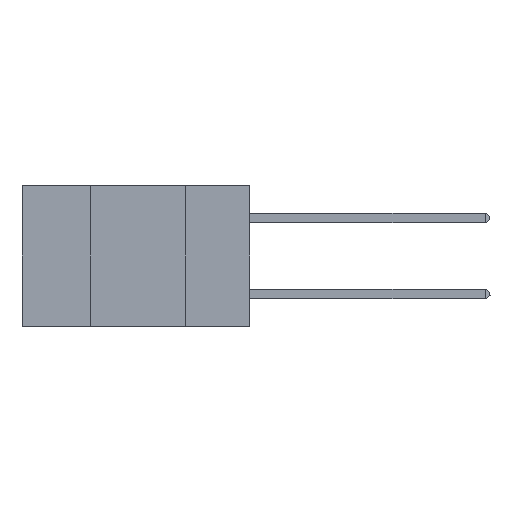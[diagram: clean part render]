
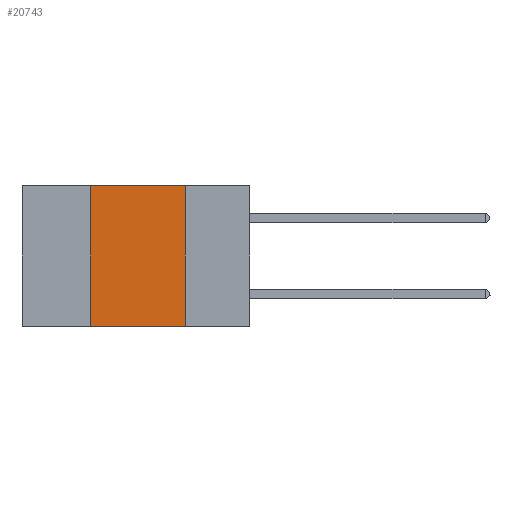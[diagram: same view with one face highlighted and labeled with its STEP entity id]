
A CAD part, left-side view. The second image highlights one B-rep face of the part: STEP entity #20743.
In plain terms, the highlighted planar face has unit normal (-1, 0, 0).
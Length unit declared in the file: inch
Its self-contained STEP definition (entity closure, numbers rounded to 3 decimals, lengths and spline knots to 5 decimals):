
#1144 = LINE ( 'NONE', #11175, #31647 ) ;
#2035 = CARTESIAN_POINT ( 'NONE',  ( 0., 0.6, 0. ) ) ;
#2526 = ORIENTED_EDGE ( 'NONE', *, *, #11613, .F. ) ;
#2671 = ORIENTED_EDGE ( 'NONE', *, *, #4228, .F. ) ;
#4228 = EDGE_CURVE ( 'NONE', #13115, #25626, #24204, .T. ) ;
#5015 = VECTOR ( 'NONE', #19980, 39.37008 ) ;
#5289 = ORIENTED_EDGE ( 'NONE', *, *, #32906, .F. ) ;
#5530 = EDGE_CURVE ( 'NONE', #36855, #7606, #1144, .T. ) ;
#5857 = EDGE_LOOP ( 'NONE', ( #2526, #2671, #5289, #28682 ) ) ;
#7606 = VERTEX_POINT ( 'NONE', #37992 ) ;
#8787 = LINE ( 'NONE', #32170, #28466 ) ;
#10577 = CARTESIAN_POINT ( 'NONE',  ( 0., 0.42, 0. ) ) ;
#11175 = CARTESIAN_POINT ( 'NONE',  ( 0., 0.6, -0.37 ) ) ;
#11613 = EDGE_CURVE ( 'NONE', #25626, #7606, #40055, .T. ) ;
#12917 = DIRECTION ( 'NONE',  ( 0., 0., 1. ) ) ;
#13115 = VERTEX_POINT ( 'NONE', #10577 ) ;
#13238 = FACE_OUTER_BOUND ( 'NONE', #5857, .T. ) ;
#13737 = VECTOR ( 'NONE', #39540, 39.37008 ) ;
#15308 = PLANE ( 'NONE',  #25705 ) ;
#17654 = DIRECTION ( 'NONE',  ( 0., -1., 0. ) ) ;
#18726 = DIRECTION ( 'NONE',  ( 1., 0., 0. ) ) ;
#19980 = DIRECTION ( 'NONE',  ( 0., 0., -1. ) ) ;
#20743 = ADVANCED_FACE ( 'NONE', ( #13238 ), #15308, .F. ) ;
#24204 = LINE ( 'NONE', #2035, #13737 ) ;
#25529 = CARTESIAN_POINT ( 'NONE',  ( 0., 0.42, -0.37 ) ) ;
#25626 = VERTEX_POINT ( 'NONE', #32098 ) ;
#25705 = AXIS2_PLACEMENT_3D ( 'NONE', #27922, #18726, #34688 ) ;
#27922 = CARTESIAN_POINT ( 'NONE',  ( 0., 0.6, 0. ) ) ;
#28466 = VECTOR ( 'NONE', #12917, 39.37008 ) ;
#28682 = ORIENTED_EDGE ( 'NONE', *, *, #5530, .T. ) ;
#29322 = CARTESIAN_POINT ( 'NONE',  ( 0., 0.17, 0. ) ) ;
#31647 = VECTOR ( 'NONE', #17654, 39.37008 ) ;
#32098 = CARTESIAN_POINT ( 'NONE',  ( 0., 0.17, 0. ) ) ;
#32170 = CARTESIAN_POINT ( 'NONE',  ( 0., 0.42, 0. ) ) ;
#32906 = EDGE_CURVE ( 'NONE', #36855, #13115, #8787, .T. ) ;
#34688 = DIRECTION ( 'NONE',  ( 0., 0., -1. ) ) ;
#36855 = VERTEX_POINT ( 'NONE', #25529 ) ;
#37992 = CARTESIAN_POINT ( 'NONE',  ( 0., 0.17, -0.37 ) ) ;
#39540 = DIRECTION ( 'NONE',  ( 0., -1., 0. ) ) ;
#40055 = LINE ( 'NONE', #29322, #5015 ) ;
